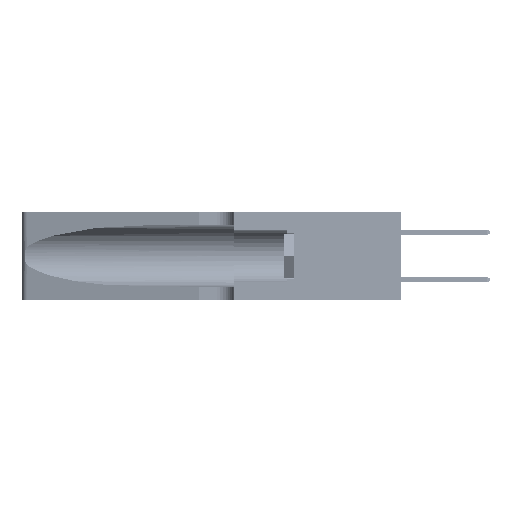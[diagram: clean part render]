
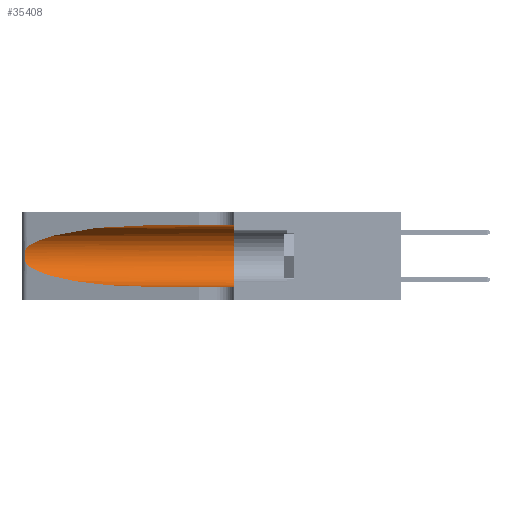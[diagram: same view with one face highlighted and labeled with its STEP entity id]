
A CAD part, left-side view. The second image highlights one B-rep face of the part: STEP entity #35408.
In plain terms, the highlighted cylindrical face has radius 3.308 mm (diameter 6.617 mm), a partial arc.
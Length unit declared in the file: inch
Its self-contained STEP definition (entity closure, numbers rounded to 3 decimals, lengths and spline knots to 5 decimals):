
#1812 = CARTESIAN_POINT ( 'NONE',  ( 0.25555, 1.22993, 0.14849 ) ) ;
#2115 = ORIENTED_EDGE ( 'NONE', *, *, #29134, .T. ) ;
#3375 = CARTESIAN_POINT ( 'NONE',  ( 0.2373, 1.15595, 0.28018 ) ) ;
#5018 = CARTESIAN_POINT ( 'NONE',  ( 0.1305, 0.35, 0.31525 ) ) ;
#5071 = EDGE_CURVE ( 'NONE', #44018, #24054, #26779, .T. ) ;
#5303 = EDGE_CURVE ( 'NONE', #17103, #44945, #28708, .T. ) ;
#5341 = EDGE_CURVE ( 'NONE', #44945, #44018, #19604, .T. ) ;
#5663 = CARTESIAN_POINT ( 'NONE',  ( 0.25639, 1.23184, 0.21858 ) ) ;
#6008 = CARTESIAN_POINT ( 'NONE',  ( 0.2373, 1.15595, 0.08982 ) ) ;
#6154 = CARTESIAN_POINT ( 'NONE',  ( 0.25487, 1.22718, 0.14631 ) ) ;
#7513 = EDGE_CURVE ( 'NONE', #24080, #24362, #25231, .T. ) ;
#8318 = CARTESIAN_POINT ( 'NONE',  ( 0.1305, 1.61858, 0.05475 ) ) ;
#8929 = CARTESIAN_POINT ( 'NONE',  ( 0.25487, 1.22718, 0.22369 ) ) ;
#9685 = CARTESIAN_POINT ( 'NONE',  ( 0.25787, 1.23484, 0.2124 ) ) ;
#13656 = CARTESIAN_POINT ( 'NONE',  ( 0.26018, 1.23835, 0.19895 ) ) ;
#14270 = DIRECTION ( 'NONE',  ( 0., -1., 0. ) ) ;
#17103 = VERTEX_POINT ( 'NONE', #8929 ) ;
#17592 = CARTESIAN_POINT ( 'NONE',  ( 0.26075, 1.23896, 0.178 ) ) ;
#17647 = AXIS2_PLACEMENT_3D ( 'NONE', #29995, #14270, #22138 ) ;
#17913 = CARTESIAN_POINT ( 'NONE',  ( 0.1305, 0.72297, 0.05475 ) ) ;
#19604 =( BOUNDED_CURVE ( )  B_SPLINE_CURVE ( 3, ( #33484, #6008, #41302, #17913 ),
 .UNSPECIFIED., .F., .F. ) 
 B_SPLINE_CURVE_WITH_KNOTS ( ( 4, 4 ),
 ( 3.44316, 4.71239 ),
 .UNSPECIFIED. ) 
 CURVE ( )  GEOMETRIC_REPRESENTATION_ITEM ( )  RATIONAL_B_SPLINE_CURVE ( ( 1., 0.87, 0.87, 1. ) ) 
 REPRESENTATION_ITEM ( '' )  );
#20355 = CARTESIAN_POINT ( 'NONE',  ( 0.1305, 0.35, 0.185 ) ) ;
#20856 = DIRECTION ( 'NONE',  ( 0., -1., 0. ) ) ;
#21343 = ORIENTED_EDGE ( 'NONE', *, *, #5071, .T. ) ;
#21375 = CARTESIAN_POINT ( 'NONE',  ( 0.25487, 1.22718, 0.22369 ) ) ;
#21532 = CARTESIAN_POINT ( 'NONE',  ( 0.25856, 1.23593, 0.16098 ) ) ;
#22138 = DIRECTION ( 'NONE',  ( 0., 0., -1. ) ) ;
#22766 = CARTESIAN_POINT ( 'NONE',  ( 0.1305, 0.35, 0.05475 ) ) ;
#23065 = CARTESIAN_POINT ( 'NONE',  ( 0.1305, 0.72297, 0.31525 ) ) ;
#23317 = EDGE_LOOP ( 'NONE', ( #2115, #23378, #24812, #21343, #43404, #38063 ) ) ;
#23378 = ORIENTED_EDGE ( 'NONE', *, *, #5303, .T. ) ;
#23673 = FACE_OUTER_BOUND ( 'NONE', #23317, .T. ) ;
#24054 = VERTEX_POINT ( 'NONE', #22766 ) ;
#24080 = VERTEX_POINT ( 'NONE', #50099 ) ;
#24312 = DIRECTION ( 'NONE',  ( 0., 0., 1. ) ) ;
#24362 = VERTEX_POINT ( 'NONE', #5018 ) ;
#24812 = ORIENTED_EDGE ( 'NONE', *, *, #5341, .T. ) ;
#24938 =( BOUNDED_CURVE ( )  B_SPLINE_CURVE ( 3, ( #23065, #46487, #3375, #30925 ),
 .UNSPECIFIED., .F., .T. ) 
 B_SPLINE_CURVE_WITH_KNOTS ( ( 4, 4 ),
 ( 1.5708, 2.84003 ),
 .UNSPECIFIED. ) 
 CURVE ( )  GEOMETRIC_REPRESENTATION_ITEM ( )  RATIONAL_B_SPLINE_CURVE ( ( 1., 0.87, 0.87, 1. ) ) 
 REPRESENTATION_ITEM ( '' )  );
#25231 = LINE ( 'NONE', #44268, #44790 ) ;
#25464 = CARTESIAN_POINT ( 'NONE',  ( 0.25639, 1.23186, 0.15144 ) ) ;
#25539 = VECTOR ( 'NONE', #35706, 39.37008 ) ;
#26779 = LINE ( 'NONE', #8318, #25539 ) ;
#26954 = CIRCLE ( 'NONE', #50508, 0.13025 ) ;
#28253 = CARTESIAN_POINT ( 'NONE',  ( 0.1305, 0.72297, 0.05475 ) ) ;
#28708 = B_SPLINE_CURVE_WITH_KNOTS ( 'NONE', 3,
 ( #21375, #48702, #5663, #9685, #37033, #13656, #40954, #17592, #44940, #21532, #48872, #25464, #1812, #29398 ),
 .UNSPECIFIED., .F., .F.,
 ( 4, 2, 2, 2, 2, 2, 4 ),
 ( 0., 0.00027, 0.00053, 0.00107, 0.0016, 0.00187, 0.00214 ),
 .UNSPECIFIED. ) ;
#29134 = EDGE_CURVE ( 'NONE', #24080, #17103, #24938, .T. ) ;
#29398 = CARTESIAN_POINT ( 'NONE',  ( 0.25487, 1.22718, 0.14631 ) ) ;
#29995 = CARTESIAN_POINT ( 'NONE',  ( 0.1305, 1.61858, 0.185 ) ) ;
#30925 = CARTESIAN_POINT ( 'NONE',  ( 0.25487, 1.22718, 0.22369 ) ) ;
#32831 = CYLINDRICAL_SURFACE ( 'NONE', #17647, 0.13025 ) ;
#33484 = CARTESIAN_POINT ( 'NONE',  ( 0.25487, 1.22718, 0.14631 ) ) ;
#35408 = ADVANCED_FACE ( 'NONE', ( #23673 ), #32831, .F. ) ;
#35706 = DIRECTION ( 'NONE',  ( 0., -1., 0. ) ) ;
#37033 = CARTESIAN_POINT ( 'NONE',  ( 0.25854, 1.2359, 0.20912 ) ) ;
#38063 = ORIENTED_EDGE ( 'NONE', *, *, #7513, .F. ) ;
#40954 = CARTESIAN_POINT ( 'NONE',  ( 0.26075, 1.23896, 0.19203 ) ) ;
#41302 = CARTESIAN_POINT ( 'NONE',  ( 0.18966, 0.96281, 0.05475 ) ) ;
#43404 = ORIENTED_EDGE ( 'NONE', *, *, #46887, .F. ) ;
#44018 = VERTEX_POINT ( 'NONE', #28253 ) ;
#44268 = CARTESIAN_POINT ( 'NONE',  ( 0.1305, 1.61858, 0.31525 ) ) ;
#44790 = VECTOR ( 'NONE', #20856, 39.37008 ) ;
#44940 = CARTESIAN_POINT ( 'NONE',  ( 0.26017, 1.23833, 0.17102 ) ) ;
#44945 = VERTEX_POINT ( 'NONE', #6154 ) ;
#46487 = CARTESIAN_POINT ( 'NONE',  ( 0.18966, 0.96281, 0.31525 ) ) ;
#46887 = EDGE_CURVE ( 'NONE', #24362, #24054, #26954, .T. ) ;
#47720 = DIRECTION ( 'NONE',  ( 0., 1., 0. ) ) ;
#48702 = CARTESIAN_POINT ( 'NONE',  ( 0.25555, 1.22994, 0.2215 ) ) ;
#48872 = CARTESIAN_POINT ( 'NONE',  ( 0.25789, 1.23486, 0.15765 ) ) ;
#50099 = CARTESIAN_POINT ( 'NONE',  ( 0.1305, 0.72297, 0.31525 ) ) ;
#50508 = AXIS2_PLACEMENT_3D ( 'NONE', #20355, #47720, #24312 ) ;
